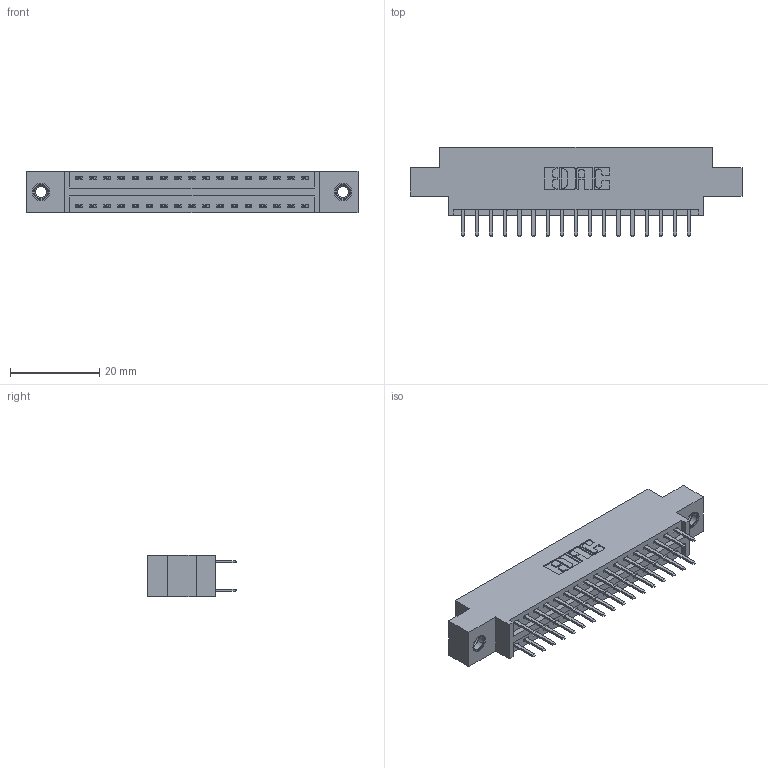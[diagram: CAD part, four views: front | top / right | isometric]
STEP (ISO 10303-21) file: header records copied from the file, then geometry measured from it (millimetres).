
FILE_DESCRIPTION (( 'STEP AP203' ), '1' );
FILE_NAME ('346-034-520-807.STEP', '2022-05-19T19:11:44', ( '' ), ( '' ), 'SwSTEP 2.0', 'SolidWorks 2020', '' );
FILE_SCHEMA (( 'CONFIG_CONTROL_DESIGN' ));
Length unit declared in the file: inch
Products named in the file (4): 346 Part_0.170 Offset - 0.156 Dia-TI; 345-250-001_345-250-005-103; 345-292-001_345-293-120; 346-034-520-807
Assembly tree (37 placements, depth 2):
  346-034-520-807
    346 Part_0.170 Offset - 0.156 Dia-TI
    345-292-001_345-293-120  x34
    345-250-001_345-250-005-103  x2
Bounding box: 74.55 x 20.02 x 9.4 mm (x, y, z)
Volume: 6892.2 mm3; surface area: 9259.2 mm2
Topology: 37 solids, 37 shells, 2090 faces, 6019 edges, 3914 vertices
Faces by surface type: plane 1370, cylinder 704, cone 12, torus 4
Entity records: 15892 total; most frequent: CARTESIAN_POINT 2651, ORIENTED_EDGE 2566, DIRECTION 2401, EDGE_CURVE 1283, VECTOR 1059, LINE 1059, VERTEX_POINT 848, AXIS2_PLACEMENT_3D 671
